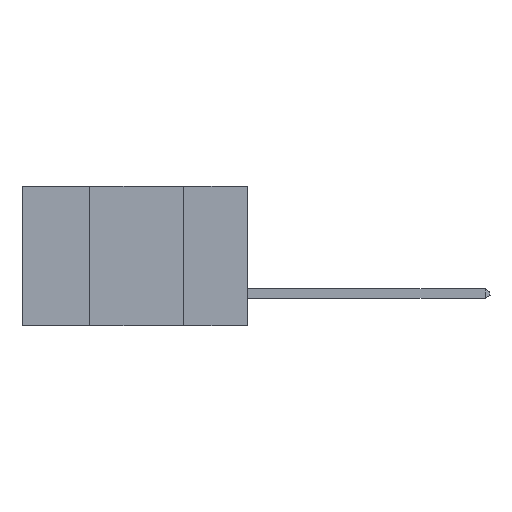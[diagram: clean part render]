
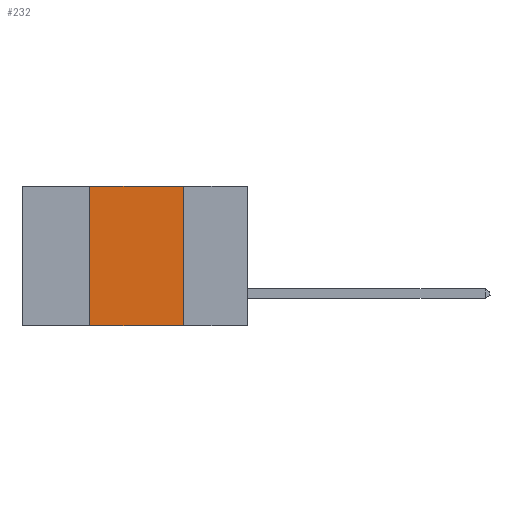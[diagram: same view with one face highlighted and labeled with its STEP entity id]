
A CAD part, left-side view. The second image highlights one B-rep face of the part: STEP entity #232.
In plain terms, the highlighted planar face has unit normal (-1, 0, 0).
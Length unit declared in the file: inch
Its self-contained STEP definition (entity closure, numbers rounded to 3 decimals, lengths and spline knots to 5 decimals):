
#232 = ADVANCED_FACE ( 'NONE', ( #8287 ), #6779, .F. ) ;
#325 = ORIENTED_EDGE ( 'NONE', *, *, #5645, .F. ) ;
#452 = CARTESIAN_POINT ( 'NONE',  ( 0., 0.42, 0. ) ) ;
#741 = EDGE_LOOP ( 'NONE', ( #1929, #325, #790, #1036 ) ) ;
#790 = ORIENTED_EDGE ( 'NONE', *, *, #10555, .F. ) ;
#1036 = ORIENTED_EDGE ( 'NONE', *, *, #7384, .T. ) ;
#1524 = DIRECTION ( 'NONE',  ( 1., 0., 0. ) ) ;
#1572 = DIRECTION ( 'NONE',  ( 0., 0., -1. ) ) ;
#1929 = ORIENTED_EDGE ( 'NONE', *, *, #10029, .F. ) ;
#2166 = LINE ( 'NONE', #3267, #4668 ) ;
#2475 = VERTEX_POINT ( 'NONE', #452 ) ;
#2837 = LINE ( 'NONE', #11405, #4164 ) ;
#3267 = CARTESIAN_POINT ( 'NONE',  ( 0., 0.42, 0. ) ) ;
#4134 = CARTESIAN_POINT ( 'NONE',  ( 0., 0.6, 0. ) ) ;
#4164 = VECTOR ( 'NONE', #5719, 39.37008 ) ;
#4478 = AXIS2_PLACEMENT_3D ( 'NONE', #4134, #1524, #1572 ) ;
#4499 = VERTEX_POINT ( 'NONE', #4560 ) ;
#4560 = CARTESIAN_POINT ( 'NONE',  ( 0., 0.17, -0.37 ) ) ;
#4668 = VECTOR ( 'NONE', #10948, 39.37008 ) ;
#5645 = EDGE_CURVE ( 'NONE', #2475, #6168, #7186, .T. ) ;
#5719 = DIRECTION ( 'NONE',  ( 0., -1., 0. ) ) ;
#6168 = VERTEX_POINT ( 'NONE', #6245 ) ;
#6245 = CARTESIAN_POINT ( 'NONE',  ( 0., 0.17, 0. ) ) ;
#6779 = PLANE ( 'NONE',  #4478 ) ;
#6789 = VECTOR ( 'NONE', #6809, 39.37008 ) ;
#6809 = DIRECTION ( 'NONE',  ( 0., 0., -1. ) ) ;
#7186 = LINE ( 'NONE', #7480, #8377 ) ;
#7384 = EDGE_CURVE ( 'NONE', #10079, #4499, #2837, .T. ) ;
#7480 = CARTESIAN_POINT ( 'NONE',  ( 0., 0.6, 0. ) ) ;
#7831 = CARTESIAN_POINT ( 'NONE',  ( 0., 0.17, 0. ) ) ;
#8287 = FACE_OUTER_BOUND ( 'NONE', #741, .T. ) ;
#8377 = VECTOR ( 'NONE', #8625, 39.37008 ) ;
#8625 = DIRECTION ( 'NONE',  ( 0., -1., 0. ) ) ;
#9163 = CARTESIAN_POINT ( 'NONE',  ( 0., 0.42, -0.37 ) ) ;
#10029 = EDGE_CURVE ( 'NONE', #6168, #4499, #11968, .T. ) ;
#10079 = VERTEX_POINT ( 'NONE', #9163 ) ;
#10555 = EDGE_CURVE ( 'NONE', #10079, #2475, #2166, .T. ) ;
#10948 = DIRECTION ( 'NONE',  ( 0., 0., 1. ) ) ;
#11405 = CARTESIAN_POINT ( 'NONE',  ( 0., 0.6, -0.37 ) ) ;
#11968 = LINE ( 'NONE', #7831, #6789 ) ;
